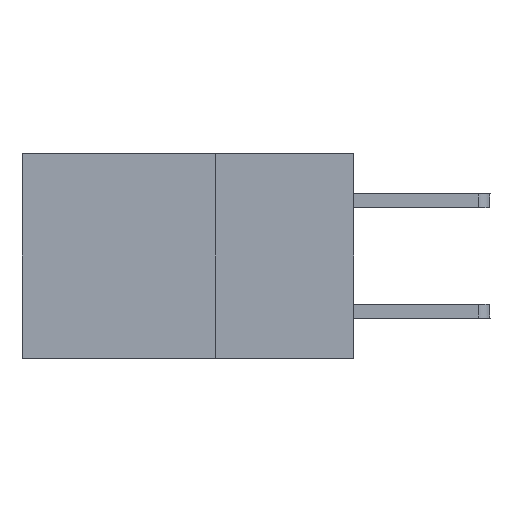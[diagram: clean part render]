
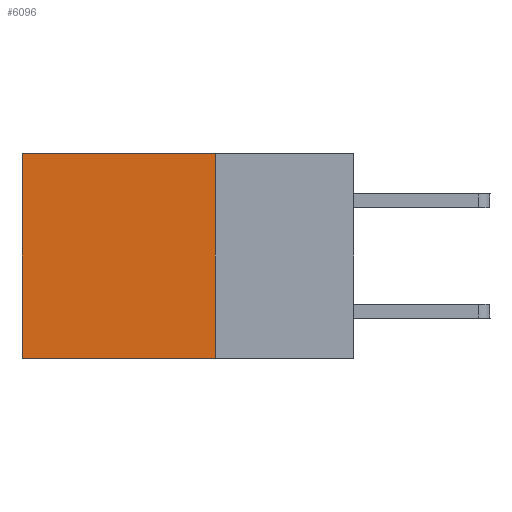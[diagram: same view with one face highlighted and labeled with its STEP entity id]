
A CAD part, left-side view. The second image highlights one B-rep face of the part: STEP entity #6096.
In plain terms, the highlighted planar face has unit normal (-1, 0, 0).
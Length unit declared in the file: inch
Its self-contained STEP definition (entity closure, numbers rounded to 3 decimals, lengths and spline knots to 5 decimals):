
#328 = DIRECTION ( 'NONE',  ( 0., 1., 0. ) ) ;
#710 = ORIENTED_EDGE ( 'NONE', *, *, #1420, .T. ) ;
#945 = CARTESIAN_POINT ( 'NONE',  ( 0.2875, 0.25, 0. ) ) ;
#946 = CARTESIAN_POINT ( 'NONE',  ( 0.2875, 0.25, 0. ) ) ;
#1420 = EDGE_CURVE ( 'NONE', #3368, #9231, #3026, .T. ) ;
#1646 = EDGE_CURVE ( 'NONE', #7672, #9231, #4151, .T. ) ;
#1719 = CARTESIAN_POINT ( 'NONE',  ( 0.2875, 0.25, 0. ) ) ;
#2103 = VECTOR ( 'NONE', #7128, 39.37008 ) ;
#2541 = CARTESIAN_POINT ( 'NONE',  ( 0.2875, 0.25, -0.37 ) ) ;
#2582 = CARTESIAN_POINT ( 'NONE',  ( 0.2875, 0.25, -0.37 ) ) ;
#3026 = LINE ( 'NONE', #8446, #7470 ) ;
#3368 = VERTEX_POINT ( 'NONE', #8680 ) ;
#3587 = ORIENTED_EDGE ( 'NONE', *, *, #9656, .T. ) ;
#3971 = LINE ( 'NONE', #946, #2103 ) ;
#4017 = DIRECTION ( 'NONE',  ( 0., 0., -1. ) ) ;
#4151 = LINE ( 'NONE', #2582, #5073 ) ;
#4153 = CARTESIAN_POINT ( 'NONE',  ( 0.2875, 0.25, 0. ) ) ;
#4566 = VERTEX_POINT ( 'NONE', #4153 ) ;
#4587 = EDGE_LOOP ( 'NONE', ( #710, #8278, #8466, #3587 ) ) ;
#4685 = CARTESIAN_POINT ( 'NONE',  ( 0.2875, 0.6, -0.37 ) ) ;
#5073 = VECTOR ( 'NONE', #328, 39.37008 ) ;
#5565 = PLANE ( 'NONE',  #7379 ) ;
#6096 = ADVANCED_FACE ( 'NONE', ( #6940 ), #5565, .F. ) ;
#6940 = FACE_OUTER_BOUND ( 'NONE', #4587, .T. ) ;
#6943 = DIRECTION ( 'NONE',  ( 0., 0., -1. ) ) ;
#7013 = DIRECTION ( 'NONE',  ( 0., 1., 0. ) ) ;
#7128 = DIRECTION ( 'NONE',  ( 0., 0., -1. ) ) ;
#7379 = AXIS2_PLACEMENT_3D ( 'NONE', #945, #8493, #4017 ) ;
#7446 = EDGE_CURVE ( 'NONE', #4566, #7672, #3971, .T. ) ;
#7470 = VECTOR ( 'NONE', #6943, 39.37008 ) ;
#7501 = VECTOR ( 'NONE', #7013, 39.37008 ) ;
#7672 = VERTEX_POINT ( 'NONE', #2541 ) ;
#7721 = LINE ( 'NONE', #1719, #7501 ) ;
#8278 = ORIENTED_EDGE ( 'NONE', *, *, #1646, .F. ) ;
#8446 = CARTESIAN_POINT ( 'NONE',  ( 0.2875, 0.6, 0. ) ) ;
#8466 = ORIENTED_EDGE ( 'NONE', *, *, #7446, .F. ) ;
#8493 = DIRECTION ( 'NONE',  ( 1., 0., 0. ) ) ;
#8680 = CARTESIAN_POINT ( 'NONE',  ( 0.2875, 0.6, 0. ) ) ;
#9231 = VERTEX_POINT ( 'NONE', #4685 ) ;
#9656 = EDGE_CURVE ( 'NONE', #4566, #3368, #7721, .T. ) ;
